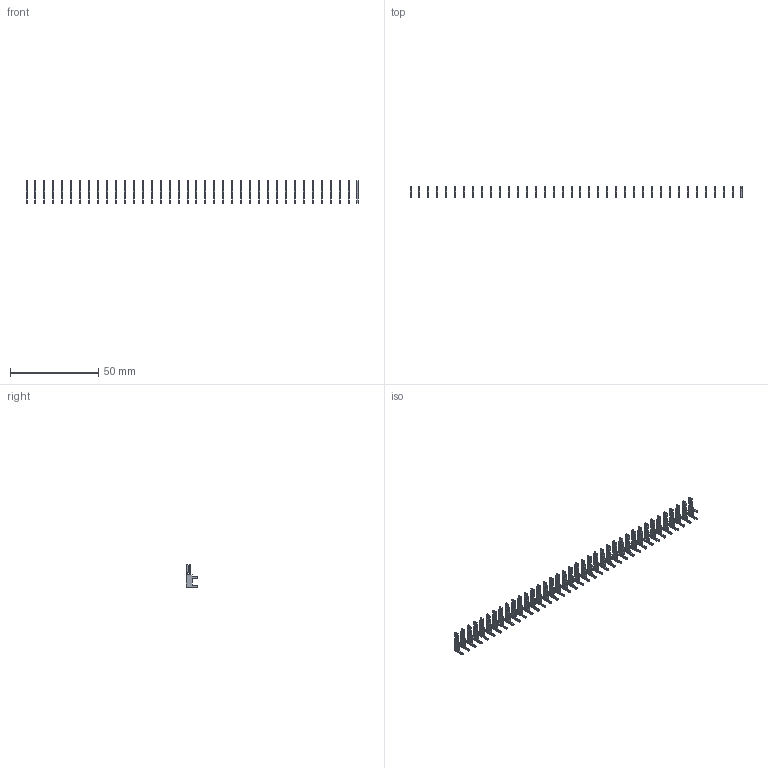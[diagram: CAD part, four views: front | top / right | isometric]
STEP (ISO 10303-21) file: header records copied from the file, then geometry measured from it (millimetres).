
FILE_DESCRIPTION (( 'STEP AP203' ), '1' );
FILE_NAME ('105-038-203-200.STEP', '2020-08-29T23:44:44', ( '' ), ( '' ), 'SwSTEP 2.0', 'SolidWorks 2020', '' );
FILE_SCHEMA (( 'CONFIG_CONTROL_DESIGN' ));
Length unit declared in the file: inch
Products named in the file (2): 100-290-001_100-290-203; 105-038-203-200
Assembly tree (38 placements, depth 2):
  105-038-203-200
    100-290-001_100-290-203  x38
Bounding box: 188.56 x 6.53 x 12.7 mm (x, y, z)
Volume: 959.3 mm3; surface area: 4397.3 mm2
Topology: 38 solids, 38 shells, 1064 faces, 2964 edges, 1976 vertices
Faces by surface type: plane 798, cylinder 266
Entity records: 2280 total; most frequent: DIRECTION 226, CARTESIAN_POINT 211, ORIENTED_EDGE 156, LOCAL_TIME 86, CALENDAR_DATE 86, COORDINATED_UNIVERSAL_TIME_OFFSET 86, DATE_AND_TIME 86, AXIS2_PLACEMENT_3D 83
